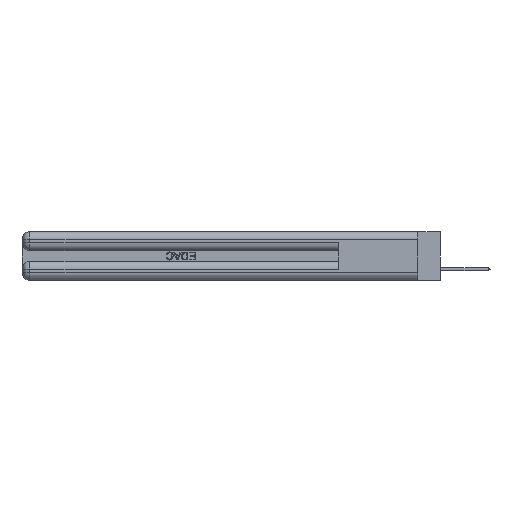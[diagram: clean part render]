
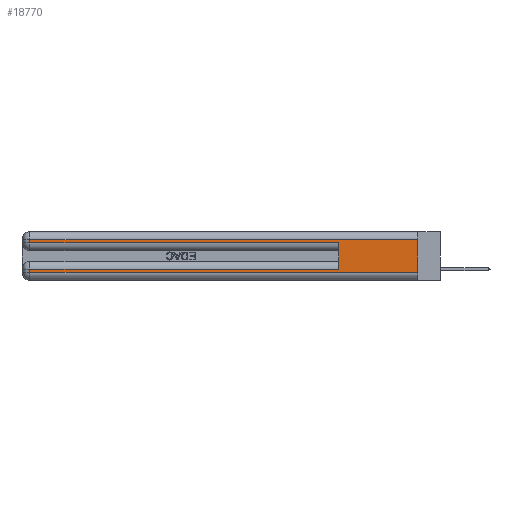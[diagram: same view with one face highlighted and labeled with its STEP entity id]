
A CAD part, left-side view. The second image highlights one B-rep face of the part: STEP entity #18770.
In plain terms, the highlighted planar face has unit normal (-1, 0, 0).
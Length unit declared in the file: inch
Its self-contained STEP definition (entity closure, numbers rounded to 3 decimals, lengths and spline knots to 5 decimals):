
#658 = CARTESIAN_POINT ( 'NONE',  ( 0., 0.6, 0.145 ) ) ;
#2068 = DIRECTION ( 'NONE',  ( 0., -1., 0. ) ) ;
#2079 = VECTOR ( 'NONE', #47602, 39.37008 ) ;
#2985 = LINE ( 'NONE', #21190, #9815 ) ;
#3336 = DIRECTION ( 'NONE',  ( 0., -1., 0. ) ) ;
#5105 = ORIENTED_EDGE ( 'NONE', *, *, #30259, .F. ) ;
#5308 = LINE ( 'NONE', #30943, #19896 ) ;
#7010 = ORIENTED_EDGE ( 'NONE', *, *, #12674, .T. ) ;
#7500 = VERTEX_POINT ( 'NONE', #52389 ) ;
#9087 = VECTOR ( 'NONE', #3336, 39.37008 ) ;
#9815 = VECTOR ( 'NONE', #49702, 39.37008 ) ;
#11615 = EDGE_CURVE ( 'NONE', #15884, #20148, #11769, .T. ) ;
#11769 = LINE ( 'NONE', #35412, #22515 ) ;
#12622 = EDGE_CURVE ( 'NONE', #7500, #18263, #5308, .T. ) ;
#12674 = EDGE_CURVE ( 'NONE', #39053, #47943, #30698, .T. ) ;
#12717 = VECTOR ( 'NONE', #42263, 39.37008 ) ;
#13507 = EDGE_CURVE ( 'NONE', #20148, #7500, #39432, .T. ) ;
#14310 = EDGE_CURVE ( 'NONE', #15884, #47943, #31816, .T. ) ;
#14316 = ORIENTED_EDGE ( 'NONE', *, *, #12622, .T. ) ;
#14938 = DIRECTION ( 'NONE',  ( 0., 0., 1. ) ) ;
#15135 = EDGE_CURVE ( 'NONE', #30572, #51669, #44938, .T. ) ;
#15884 = VERTEX_POINT ( 'NONE', #41283 ) ;
#16521 = CARTESIAN_POINT ( 'NONE',  ( 0., 2.94, 0.085 ) ) ;
#18263 = VERTEX_POINT ( 'NONE', #36625 ) ;
#18770 = ADVANCED_FACE ( 'NONE', ( #43476 ), #51383, .F. ) ;
#19631 = ORIENTED_EDGE ( 'NONE', *, *, #14310, .F. ) ;
#19896 = VECTOR ( 'NONE', #2068, 39.37008 ) ;
#20148 = VERTEX_POINT ( 'NONE', #16521 ) ;
#21190 = CARTESIAN_POINT ( 'NONE',  ( 0., 0., 0.37 ) ) ;
#21770 = AXIS2_PLACEMENT_3D ( 'NONE', #32464, #32135, #23958 ) ;
#22420 = DIRECTION ( 'NONE',  ( 0., 1., 0. ) ) ;
#22515 = VECTOR ( 'NONE', #26710, 39.37008 ) ;
#22797 = VECTOR ( 'NONE', #22420, 39.37008 ) ;
#23958 = DIRECTION ( 'NONE',  ( 0., 0., -1. ) ) ;
#24158 = VECTOR ( 'NONE', #14938, 39.37008 ) ;
#26036 = ORIENTED_EDGE ( 'NONE', *, *, #13507, .T. ) ;
#26710 = DIRECTION ( 'NONE',  ( 0., 1., 0. ) ) ;
#27061 = CARTESIAN_POINT ( 'NONE',  ( 0., 2.94, 0.37 ) ) ;
#30259 = EDGE_CURVE ( 'NONE', #30572, #18263, #2985, .T. ) ;
#30572 = VERTEX_POINT ( 'NONE', #45470 ) ;
#30698 = LINE ( 'NONE', #31262, #9087 ) ;
#30943 = CARTESIAN_POINT ( 'NONE',  ( 0., 0., 0.06 ) ) ;
#31262 = CARTESIAN_POINT ( 'NONE',  ( 0., 0., 0.285 ) ) ;
#31816 = LINE ( 'NONE', #658, #24158 ) ;
#32135 = DIRECTION ( 'NONE',  ( 1., 0., 0. ) ) ;
#32464 = CARTESIAN_POINT ( 'NONE',  ( 0., 0., 0.37 ) ) ;
#32837 = CARTESIAN_POINT ( 'NONE',  ( 0., 2.94, 0.31 ) ) ;
#34310 = LINE ( 'NONE', #37489, #12717 ) ;
#35412 = CARTESIAN_POINT ( 'NONE',  ( 0., 0., 0.085 ) ) ;
#35484 = ORIENTED_EDGE ( 'NONE', *, *, #11615, .T. ) ;
#35809 = CARTESIAN_POINT ( 'NONE',  ( 0., 0.6, 0.285 ) ) ;
#36625 = CARTESIAN_POINT ( 'NONE',  ( 0., 0., 0.06 ) ) ;
#37489 = CARTESIAN_POINT ( 'NONE',  ( 0., 2.94, 0.37 ) ) ;
#38458 = ORIENTED_EDGE ( 'NONE', *, *, #49539, .T. ) ;
#39053 = VERTEX_POINT ( 'NONE', #47684 ) ;
#39432 = LINE ( 'NONE', #27061, #2079 ) ;
#41283 = CARTESIAN_POINT ( 'NONE',  ( 0., 0.6, 0.085 ) ) ;
#42263 = DIRECTION ( 'NONE',  ( 0., 0., -1. ) ) ;
#42264 = CARTESIAN_POINT ( 'NONE',  ( 0., 0., 0.31 ) ) ;
#42970 = ORIENTED_EDGE ( 'NONE', *, *, #15135, .T. ) ;
#43476 = FACE_OUTER_BOUND ( 'NONE', #51640, .T. ) ;
#44938 = LINE ( 'NONE', #42264, #22797 ) ;
#45470 = CARTESIAN_POINT ( 'NONE',  ( 0., 0., 0.31 ) ) ;
#47602 = DIRECTION ( 'NONE',  ( 0., 0., -1. ) ) ;
#47684 = CARTESIAN_POINT ( 'NONE',  ( 0., 2.94, 0.285 ) ) ;
#47943 = VERTEX_POINT ( 'NONE', #35809 ) ;
#49539 = EDGE_CURVE ( 'NONE', #51669, #39053, #34310, .T. ) ;
#49702 = DIRECTION ( 'NONE',  ( 0., 0., -1. ) ) ;
#51383 = PLANE ( 'NONE',  #21770 ) ;
#51640 = EDGE_LOOP ( 'NONE', ( #5105, #42970, #38458, #7010, #19631, #35484, #26036, #14316 ) ) ;
#51669 = VERTEX_POINT ( 'NONE', #32837 ) ;
#52389 = CARTESIAN_POINT ( 'NONE',  ( 0., 2.94, 0.06 ) ) ;
